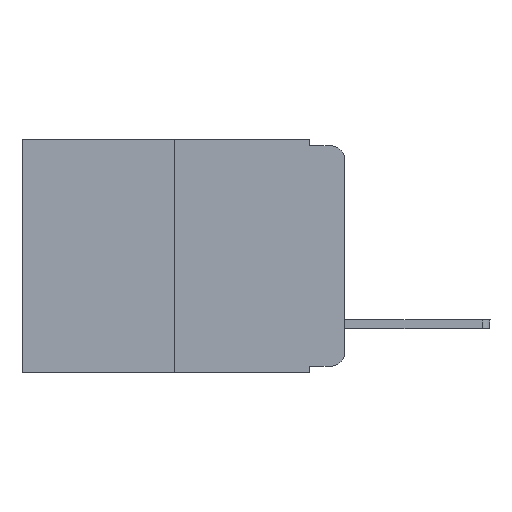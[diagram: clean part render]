
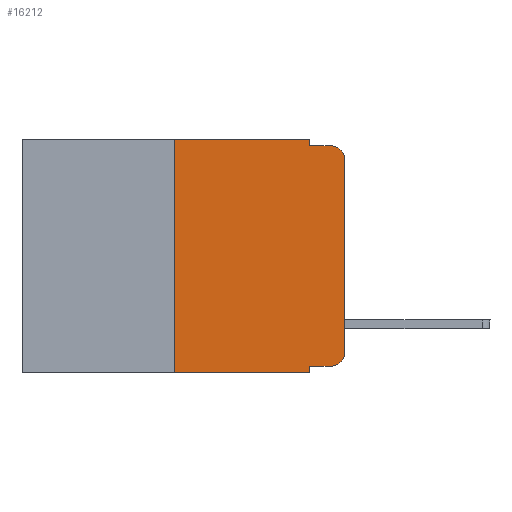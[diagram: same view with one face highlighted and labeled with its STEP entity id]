
A CAD part, left-side view. The second image highlights one B-rep face of the part: STEP entity #16212.
In plain terms, the highlighted planar face has unit normal (-1, 0, 0).
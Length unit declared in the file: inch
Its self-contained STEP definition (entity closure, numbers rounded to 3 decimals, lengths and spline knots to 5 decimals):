
#274 = AXIS2_PLACEMENT_3D ( 'NONE', #446, #3303, #10400 ) ;
#276 = DIRECTION ( 'NONE',  ( 0., 0., -1. ) ) ;
#307 = ORIENTED_EDGE ( 'NONE', *, *, #9285, .F. ) ;
#446 = CARTESIAN_POINT ( 'NONE',  ( 0., 0.473, 0. ) ) ;
#517 = DIRECTION ( 'NONE',  ( -1., 0., 0. ) ) ;
#524 = LINE ( 'NONE', #1487, #13897 ) ;
#529 = ORIENTED_EDGE ( 'NONE', *, *, #13995, .T. ) ;
#781 = DIRECTION ( 'NONE',  ( 0., 0., -1. ) ) ;
#787 = CIRCLE ( 'NONE', #12894, 0.02 ) ;
#1082 = VECTOR ( 'NONE', #16294, 39.37008 ) ;
#1418 = CARTESIAN_POINT ( 'NONE',  ( 0., 0.473, -0.343 ) ) ;
#1487 = CARTESIAN_POINT ( 'NONE',  ( 0., 0.473, 0. ) ) ;
#1563 = ORIENTED_EDGE ( 'NONE', *, *, #10255, .F. ) ;
#1785 = VERTEX_POINT ( 'NONE', #12309 ) ;
#1951 = ORIENTED_EDGE ( 'NONE', *, *, #16041, .F. ) ;
#2729 = VERTEX_POINT ( 'NONE', #5923 ) ;
#3079 = DIRECTION ( 'NONE',  ( 0., -1., 0. ) ) ;
#3251 = VERTEX_POINT ( 'NONE', #14824 ) ;
#3256 = VERTEX_POINT ( 'NONE', #11963 ) ;
#3303 = DIRECTION ( 'NONE',  ( 1., 0., 0. ) ) ;
#3634 = CARTESIAN_POINT ( 'NONE',  ( 0., 0.051, 0. ) ) ;
#3694 = EDGE_CURVE ( 'NONE', #6849, #4669, #787, .T. ) ;
#4053 = DIRECTION ( 'NONE',  ( 0., 0., 1. ) ) ;
#4094 = EDGE_CURVE ( 'NONE', #4997, #1785, #11785, .T. ) ;
#4669 = VERTEX_POINT ( 'NONE', #10378 ) ;
#4947 = CARTESIAN_POINT ( 'NONE',  ( 0., 0.02, -0.03 ) ) ;
#4997 = VERTEX_POINT ( 'NONE', #12149 ) ;
#5105 = CIRCLE ( 'NONE', #16309, 0.02 ) ;
#5235 = VECTOR ( 'NONE', #7738, 39.37008 ) ;
#5452 = ORIENTED_EDGE ( 'NONE', *, *, #7029, .T. ) ;
#5676 = CARTESIAN_POINT ( 'NONE',  ( 0., 0.051, -0.343 ) ) ;
#5774 = VECTOR ( 'NONE', #4053, 39.37008 ) ;
#5923 = CARTESIAN_POINT ( 'NONE',  ( 0., 0., -0.03 ) ) ;
#6115 = VERTEX_POINT ( 'NONE', #16580 ) ;
#6123 = DIRECTION ( 'NONE',  ( 0., -1., 0. ) ) ;
#6131 = PLANE ( 'NONE',  #274 ) ;
#6744 = ORIENTED_EDGE ( 'NONE', *, *, #4094, .F. ) ;
#6792 = CARTESIAN_POINT ( 'NONE',  ( 0., 0.051, -0.333 ) ) ;
#6849 = VERTEX_POINT ( 'NONE', #7942 ) ;
#7029 = EDGE_CURVE ( 'NONE', #3256, #6849, #17786, .T. ) ;
#7738 = DIRECTION ( 'NONE',  ( 0., 0., -1. ) ) ;
#7920 = EDGE_CURVE ( 'NONE', #2729, #3251, #5105, .T. ) ;
#7942 = CARTESIAN_POINT ( 'NONE',  ( 0., 0.02, -0.333 ) ) ;
#8159 = LINE ( 'NONE', #9675, #5774 ) ;
#8263 = LINE ( 'NONE', #1418, #11528 ) ;
#8586 = EDGE_LOOP ( 'NONE', ( #16163, #8842, #1563, #6744, #1951, #307, #529, #8596, #5452, #12472 ) ) ;
#8596 = ORIENTED_EDGE ( 'NONE', *, *, #10284, .F. ) ;
#8842 = ORIENTED_EDGE ( 'NONE', *, *, #7920, .T. ) ;
#9141 = DIRECTION ( 'NONE',  ( -1., 0., 0. ) ) ;
#9285 = EDGE_CURVE ( 'NONE', #15922, #6115, #10726, .T. ) ;
#9675 = CARTESIAN_POINT ( 'NONE',  ( 0., 0., 0. ) ) ;
#10095 = VECTOR ( 'NONE', #3079, 39.37008 ) ;
#10255 = EDGE_CURVE ( 'NONE', #1785, #3251, #16190, .T. ) ;
#10284 = EDGE_CURVE ( 'NONE', #3256, #14947, #17266, .T. ) ;
#10292 = CARTESIAN_POINT ( 'NONE',  ( 0., 0.02, -0.313 ) ) ;
#10378 = CARTESIAN_POINT ( 'NONE',  ( 0., 0., -0.313 ) ) ;
#10400 = DIRECTION ( 'NONE',  ( 0., 0., -1. ) ) ;
#10726 = LINE ( 'NONE', #17818, #1082 ) ;
#11486 = VECTOR ( 'NONE', #6123, 39.37008 ) ;
#11528 = VECTOR ( 'NONE', #16739, 39.37008 ) ;
#11702 = DIRECTION ( 'NONE',  ( 0., 0., -1. ) ) ;
#11785 = LINE ( 'NONE', #3634, #5235 ) ;
#11963 = CARTESIAN_POINT ( 'NONE',  ( 0., 0.051, -0.333 ) ) ;
#12149 = CARTESIAN_POINT ( 'NONE',  ( 0., 0.051, 0. ) ) ;
#12309 = CARTESIAN_POINT ( 'NONE',  ( 0., 0.051, -0.01 ) ) ;
#12472 = ORIENTED_EDGE ( 'NONE', *, *, #3694, .T. ) ;
#12894 = AXIS2_PLACEMENT_3D ( 'NONE', #10292, #517, #11702 ) ;
#12930 = DIRECTION ( 'NONE',  ( 0., -1., 0. ) ) ;
#13897 = VECTOR ( 'NONE', #12930, 39.37008 ) ;
#13995 = EDGE_CURVE ( 'NONE', #15922, #14947, #8263, .T. ) ;
#14112 = CARTESIAN_POINT ( 'NONE',  ( 0., 0.051, -0.01 ) ) ;
#14824 = CARTESIAN_POINT ( 'NONE',  ( 0., 0.02, -0.01 ) ) ;
#14947 = VERTEX_POINT ( 'NONE', #5676 ) ;
#15392 = FACE_OUTER_BOUND ( 'NONE', #8586, .T. ) ;
#15663 = CARTESIAN_POINT ( 'NONE',  ( 0., 0.051, 0. ) ) ;
#15922 = VERTEX_POINT ( 'NONE', #17250 ) ;
#16041 = EDGE_CURVE ( 'NONE', #6115, #4997, #524, .T. ) ;
#16163 = ORIENTED_EDGE ( 'NONE', *, *, #16696, .T. ) ;
#16190 = LINE ( 'NONE', #14112, #10095 ) ;
#16212 = ADVANCED_FACE ( 'NONE', ( #15392 ), #6131, .F. ) ;
#16294 = DIRECTION ( 'NONE',  ( 0., 0., 1. ) ) ;
#16309 = AXIS2_PLACEMENT_3D ( 'NONE', #4947, #9141, #781 ) ;
#16580 = CARTESIAN_POINT ( 'NONE',  ( 0., 0.25, 0. ) ) ;
#16696 = EDGE_CURVE ( 'NONE', #4669, #2729, #8159, .T. ) ;
#16739 = DIRECTION ( 'NONE',  ( 0., -1., 0. ) ) ;
#17250 = CARTESIAN_POINT ( 'NONE',  ( 0., 0.25, -0.343 ) ) ;
#17266 = LINE ( 'NONE', #15663, #17719 ) ;
#17719 = VECTOR ( 'NONE', #276, 39.37008 ) ;
#17786 = LINE ( 'NONE', #6792, #11486 ) ;
#17818 = CARTESIAN_POINT ( 'NONE',  ( 0., 0.25, 0. ) ) ;
